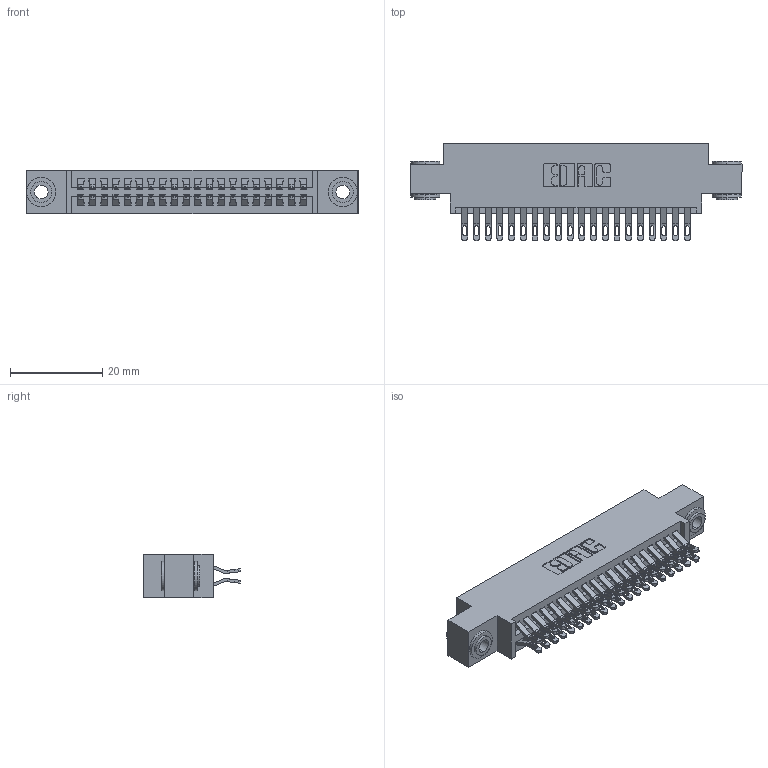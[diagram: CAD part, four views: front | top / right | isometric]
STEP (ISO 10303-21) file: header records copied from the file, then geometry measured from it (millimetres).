
FILE_DESCRIPTION (( 'STEP AP203' ), '1' );
FILE_NAME ('395-040-555-803.STEP', '2019-10-18T05:51:50', ( '' ), ( '' ), 'SwSTEP 2.0', 'SolidWorks 2016', '' );
FILE_SCHEMA (( 'CONFIG_CONTROL_DESIGN' ));
Length unit declared in the file: inch
Products named in the file (4): 345 Part_0.170 Offset - 0.156 Dia-TH; 345-292-001_555 Tail; 345-250-002_345-250-002-102; 395-040-555-803
Assembly tree (43 placements, depth 2):
  395-040-555-803
    345 Part_0.170 Offset - 0.156 Dia-TH
    345-292-001_555 Tail  x40
    345-250-002_345-250-002-102  x2
Bounding box: 72.01 x 21.13 x 9.4 mm (x, y, z)
Volume: 6812.8 mm3; surface area: 10396.3 mm2
Topology: 43 solids, 43 shells, 2408 faces, 7509 edges, 5002 vertices
Faces by surface type: plane 1334, cylinder 1066, cone 8
Entity records: 19762 total; most frequent: CARTESIAN_POINT 3345, ORIENTED_EDGE 3242, DIRECTION 2975, EDGE_CURVE 1621, VECTOR 1365, LINE 1365, VERTEX_POINT 1078, AXIS2_PLACEMENT_3D 805
